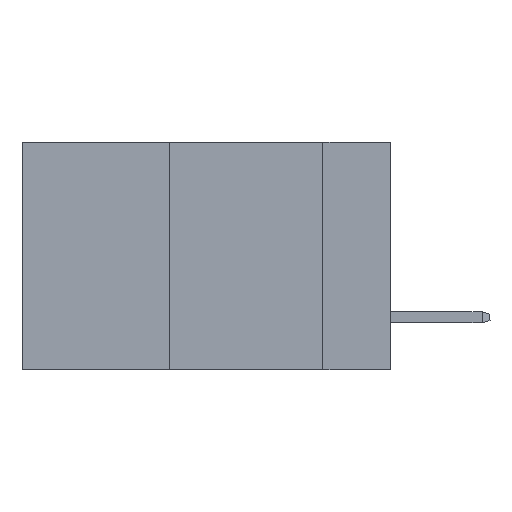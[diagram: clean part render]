
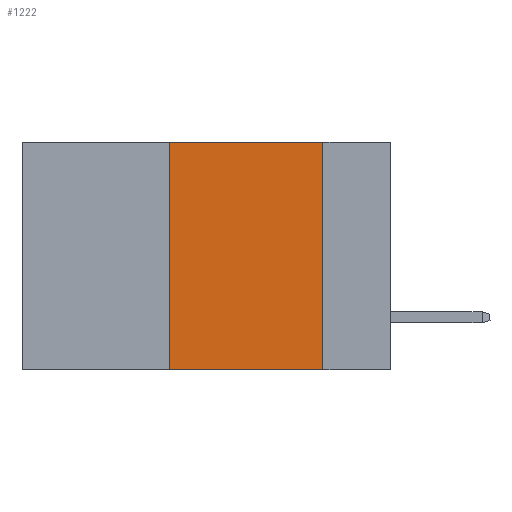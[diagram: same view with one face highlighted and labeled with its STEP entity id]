
A CAD part, left-side view. The second image highlights one B-rep face of the part: STEP entity #1222.
In plain terms, the highlighted planar face has unit normal (-1, 0, 0).
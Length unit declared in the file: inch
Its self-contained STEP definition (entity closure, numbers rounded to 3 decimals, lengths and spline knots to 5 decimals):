
#76 = EDGE_LOOP ( 'NONE', ( #9742, #4818, #7673, #10758 ) ) ;
#583 = PLANE ( 'NONE',  #844 ) ;
#746 = CARTESIAN_POINT ( 'NONE',  ( 0., 0.6, 0. ) ) ;
#844 = AXIS2_PLACEMENT_3D ( 'NONE', #6283, #2056, #1971 ) ;
#1168 = DIRECTION ( 'NONE',  ( 0., -1., 0. ) ) ;
#1222 = ADVANCED_FACE ( 'NONE', ( #11508 ), #583, .F. ) ;
#1290 = LINE ( 'NONE', #4112, #11797 ) ;
#1519 = EDGE_CURVE ( 'NONE', #6898, #4117, #10719, .T. ) ;
#1971 = DIRECTION ( 'NONE',  ( 0., 0., -1. ) ) ;
#2056 = DIRECTION ( 'NONE',  ( 1., 0., 0. ) ) ;
#2224 = CARTESIAN_POINT ( 'NONE',  ( 0., 0.11, 0. ) ) ;
#2456 = VECTOR ( 'NONE', #9921, 39.37008 ) ;
#3614 = EDGE_CURVE ( 'NONE', #4117, #5262, #7910, .T. ) ;
#4112 = CARTESIAN_POINT ( 'NONE',  ( 0., 0.36, 0. ) ) ;
#4117 = VERTEX_POINT ( 'NONE', #2224 ) ;
#4491 = EDGE_CURVE ( 'NONE', #4632, #5262, #7753, .T. ) ;
#4570 = CARTESIAN_POINT ( 'NONE',  ( 0., 0.11, -0.37 ) ) ;
#4632 = VERTEX_POINT ( 'NONE', #9257 ) ;
#4818 = ORIENTED_EDGE ( 'NONE', *, *, #1519, .F. ) ;
#5262 = VERTEX_POINT ( 'NONE', #4570 ) ;
#6283 = CARTESIAN_POINT ( 'NONE',  ( 0., 0.6, 0. ) ) ;
#6898 = VERTEX_POINT ( 'NONE', #9851 ) ;
#7673 = ORIENTED_EDGE ( 'NONE', *, *, #13114, .F. ) ;
#7753 = LINE ( 'NONE', #10799, #10046 ) ;
#7910 = LINE ( 'NONE', #13146, #2456 ) ;
#9257 = CARTESIAN_POINT ( 'NONE',  ( 0., 0.36, -0.37 ) ) ;
#9742 = ORIENTED_EDGE ( 'NONE', *, *, #3614, .F. ) ;
#9851 = CARTESIAN_POINT ( 'NONE',  ( 0., 0.36, 0. ) ) ;
#9921 = DIRECTION ( 'NONE',  ( 0., 0., -1. ) ) ;
#10046 = VECTOR ( 'NONE', #10501, 39.37008 ) ;
#10501 = DIRECTION ( 'NONE',  ( 0., -1., 0. ) ) ;
#10719 = LINE ( 'NONE', #746, #13037 ) ;
#10758 = ORIENTED_EDGE ( 'NONE', *, *, #4491, .T. ) ;
#10799 = CARTESIAN_POINT ( 'NONE',  ( 0., 0.6, -0.37 ) ) ;
#11508 = FACE_OUTER_BOUND ( 'NONE', #76, .T. ) ;
#11797 = VECTOR ( 'NONE', #13100, 39.37008 ) ;
#13037 = VECTOR ( 'NONE', #1168, 39.37008 ) ;
#13100 = DIRECTION ( 'NONE',  ( 0., 0., 1. ) ) ;
#13114 = EDGE_CURVE ( 'NONE', #4632, #6898, #1290, .T. ) ;
#13146 = CARTESIAN_POINT ( 'NONE',  ( 0., 0.11, 0. ) ) ;
